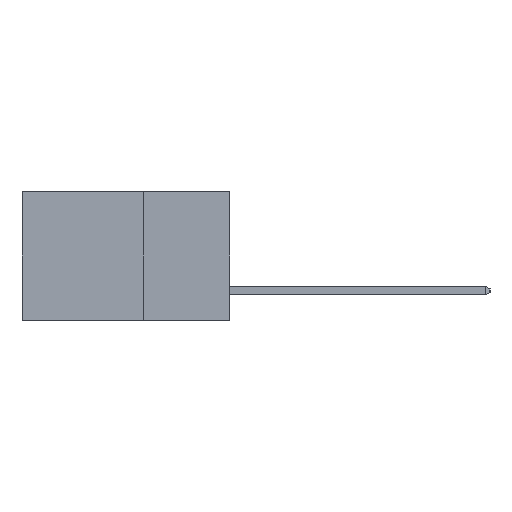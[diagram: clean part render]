
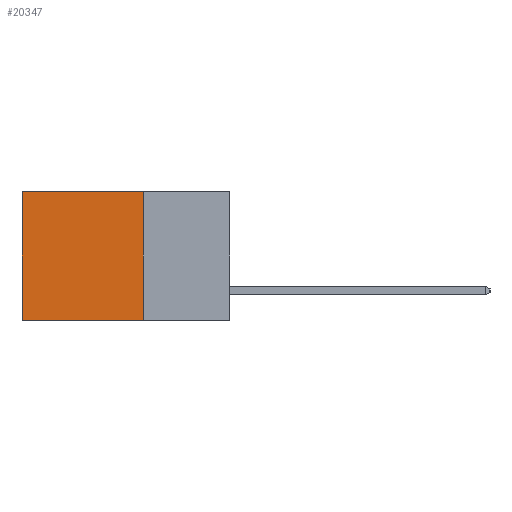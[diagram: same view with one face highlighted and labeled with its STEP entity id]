
A CAD part, left-side view. The second image highlights one B-rep face of the part: STEP entity #20347.
In plain terms, the highlighted planar face has unit normal (-1, 0, 0).
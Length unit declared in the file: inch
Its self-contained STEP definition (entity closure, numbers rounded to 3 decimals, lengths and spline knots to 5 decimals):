
#96 = CARTESIAN_POINT ( 'NONE',  ( 0.298, 0.25, 0. ) ) ;
#765 = DIRECTION ( 'NONE',  ( 0., 1., 0. ) ) ;
#1100 = VERTEX_POINT ( 'NONE', #5902 ) ;
#2081 = DIRECTION ( 'NONE',  ( 0., 0., -1. ) ) ;
#2607 = CARTESIAN_POINT ( 'NONE',  ( 0.298, 0.25, 0. ) ) ;
#2927 = CARTESIAN_POINT ( 'NONE',  ( 0.298, 0.25, -0.37 ) ) ;
#3576 = LINE ( 'NONE', #11042, #7908 ) ;
#4079 = EDGE_CURVE ( 'NONE', #13477, #14352, #6955, .T. ) ;
#5902 = CARTESIAN_POINT ( 'NONE',  ( 0.298, 0.25, -0.37 ) ) ;
#6196 = ORIENTED_EDGE ( 'NONE', *, *, #23961, .F. ) ;
#6941 = EDGE_CURVE ( 'NONE', #13477, #1100, #25782, .T. ) ;
#6955 = LINE ( 'NONE', #96, #12668 ) ;
#7908 = VECTOR ( 'NONE', #25916, 39.37008 ) ;
#11036 = DIRECTION ( 'NONE',  ( 0., 1., 0. ) ) ;
#11042 = CARTESIAN_POINT ( 'NONE',  ( 0.298, 0.6, 0. ) ) ;
#11088 = ORIENTED_EDGE ( 'NONE', *, *, #6941, .F. ) ;
#11270 = CARTESIAN_POINT ( 'NONE',  ( 0.298, 0.25, 0. ) ) ;
#12668 = VECTOR ( 'NONE', #11036, 39.37008 ) ;
#12810 = EDGE_CURVE ( 'NONE', #14352, #17724, #3576, .T. ) ;
#13477 = VERTEX_POINT ( 'NONE', #2607 ) ;
#14352 = VERTEX_POINT ( 'NONE', #14643 ) ;
#14519 = VECTOR ( 'NONE', #26233, 39.37008 ) ;
#14643 = CARTESIAN_POINT ( 'NONE',  ( 0.298, 0.6, 0. ) ) ;
#14898 = DIRECTION ( 'NONE',  ( 1., 0., 0. ) ) ;
#16057 = VECTOR ( 'NONE', #765, 39.37008 ) ;
#17724 = VERTEX_POINT ( 'NONE', #26530 ) ;
#20347 = ADVANCED_FACE ( 'NONE', ( #27529 ), #23350, .F. ) ;
#20554 = ORIENTED_EDGE ( 'NONE', *, *, #4079, .T. ) ;
#21717 = LINE ( 'NONE', #2927, #16057 ) ;
#23350 = PLANE ( 'NONE',  #27311 ) ;
#23961 = EDGE_CURVE ( 'NONE', #1100, #17724, #21717, .T. ) ;
#24298 = EDGE_LOOP ( 'NONE', ( #24996, #6196, #11088, #20554 ) ) ;
#24996 = ORIENTED_EDGE ( 'NONE', *, *, #12810, .T. ) ;
#25782 = LINE ( 'NONE', #11270, #14519 ) ;
#25916 = DIRECTION ( 'NONE',  ( 0., 0., -1. ) ) ;
#26233 = DIRECTION ( 'NONE',  ( 0., 0., -1. ) ) ;
#26530 = CARTESIAN_POINT ( 'NONE',  ( 0.298, 0.6, -0.37 ) ) ;
#27311 = AXIS2_PLACEMENT_3D ( 'NONE', #27517, #14898, #2081 ) ;
#27517 = CARTESIAN_POINT ( 'NONE',  ( 0.298, 0.25, 0. ) ) ;
#27529 = FACE_OUTER_BOUND ( 'NONE', #24298, .T. ) ;
